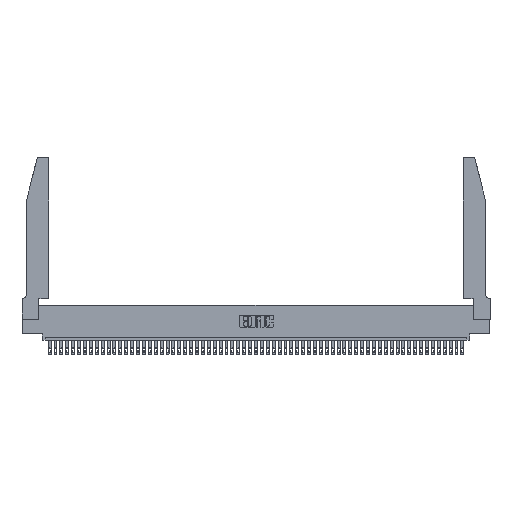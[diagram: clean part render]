
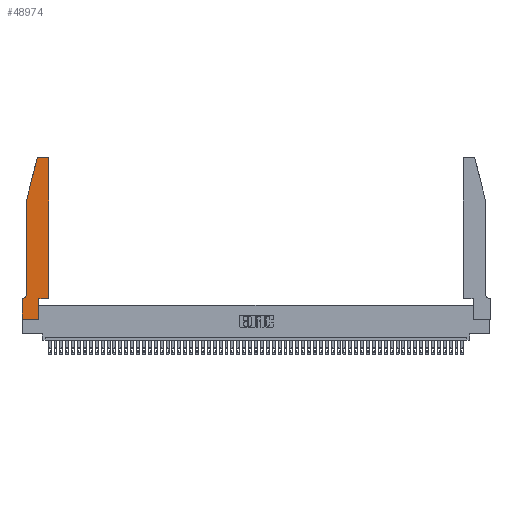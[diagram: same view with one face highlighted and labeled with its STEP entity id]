
A CAD part, top view. The second image highlights one B-rep face of the part: STEP entity #48974.
In plain terms, the highlighted planar face has unit normal (0, 0, 1).
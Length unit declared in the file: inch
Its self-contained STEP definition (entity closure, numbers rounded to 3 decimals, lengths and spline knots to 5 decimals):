
#235 = LINE ( 'NONE', #23584, #13973 ) ;
#309 = ORIENTED_EDGE ( 'NONE', *, *, #26216, .T. ) ;
#399 = LINE ( 'NONE', #14041, #47661 ) ;
#977 = EDGE_CURVE ( 'NONE', #34113, #47304, #235, .T. ) ;
#1268 = DIRECTION ( 'NONE',  ( 0., -1., 0. ) ) ;
#1806 = CIRCLE ( 'NONE', #15870, 0.07 ) ;
#2004 = DIRECTION ( 'NONE',  ( -1., 0., 0. ) ) ;
#3105 = LINE ( 'NONE', #48498, #46448 ) ;
#3688 = DIRECTION ( 'NONE',  ( 1., 0., 0. ) ) ;
#4073 = CARTESIAN_POINT ( 'NONE',  ( 0.4505, 2.72, 0.37 ) ) ;
#5131 = ORIENTED_EDGE ( 'NONE', *, *, #16956, .T. ) ;
#5728 = DIRECTION ( 'NONE',  ( 0., 0., 1. ) ) ;
#6964 = VERTEX_POINT ( 'NONE', #10926 ) ;
#7626 = ORIENTED_EDGE ( 'NONE', *, *, #21330, .T. ) ;
#7640 = EDGE_CURVE ( 'NONE', #53000, #34113, #32343, .T. ) ;
#10670 = VECTOR ( 'NONE', #36656, 39.37008 ) ;
#10926 = CARTESIAN_POINT ( 'NONE',  ( 0.0755, 0.42, 0.37 ) ) ;
#11258 = CARTESIAN_POINT ( 'NONE',  ( 0., 0., 0.37 ) ) ;
#11355 = CARTESIAN_POINT ( 'NONE',  ( 0., 0., 0.37 ) ) ;
#12174 = CARTESIAN_POINT ( 'NONE',  ( 0.4205, 2.72, 0.37 ) ) ;
#13198 = ORIENTED_EDGE ( 'NONE', *, *, #43641, .T. ) ;
#13973 = VECTOR ( 'NONE', #48124, 39.37008 ) ;
#14041 = CARTESIAN_POINT ( 'NONE',  ( 0., 0., 0.37 ) ) ;
#14532 = VECTOR ( 'NONE', #49606, 39.37008 ) ;
#15870 = AXIS2_PLACEMENT_3D ( 'NONE', #52650, #45582, #28115 ) ;
#16956 = EDGE_CURVE ( 'NONE', #47304, #45289, #17943, .T. ) ;
#17035 = ORIENTED_EDGE ( 'NONE', *, *, #7640, .T. ) ;
#17943 = LINE ( 'NONE', #32434, #42941 ) ;
#19148 = CARTESIAN_POINT ( 'NONE',  ( 0.0755, 2., 0.37 ) ) ;
#20047 = EDGE_CURVE ( 'NONE', #6964, #53029, #1806, .T. ) ;
#20269 = ORIENTED_EDGE ( 'NONE', *, *, #977, .T. ) ;
#20418 = DIRECTION ( 'NONE',  ( 1., 0., 0. ) ) ;
#20957 = CARTESIAN_POINT ( 'NONE',  ( 0., 0.35, 0.37 ) ) ;
#21146 = VECTOR ( 'NONE', #40324, 39.37008 ) ;
#21330 = EDGE_CURVE ( 'NONE', #27046, #53000, #399, .T. ) ;
#21798 = LINE ( 'NONE', #47888, #10670 ) ;
#21905 = DIRECTION ( 'NONE',  ( -0.239, -0.971, 0. ) ) ;
#23169 = CARTESIAN_POINT ( 'NONE',  ( 0.0755, 0.35, 0.37 ) ) ;
#23584 = CARTESIAN_POINT ( 'NONE',  ( 0.2865, 0.35, 0.37 ) ) ;
#24395 = CIRCLE ( 'NONE', #32426, 0.03 ) ;
#24747 = VECTOR ( 'NONE', #21905, 39.37008 ) ;
#24847 = EDGE_CURVE ( 'NONE', #53029, #27046, #38065, .T. ) ;
#25334 = VERTEX_POINT ( 'NONE', #4073 ) ;
#26216 = EDGE_CURVE ( 'NONE', #31813, #6964, #3105, .T. ) ;
#26396 = CARTESIAN_POINT ( 'NONE',  ( 0.284, 2.75, 0.37 ) ) ;
#26504 = ORIENTED_EDGE ( 'NONE', *, *, #39388, .T. ) ;
#27046 = VERTEX_POINT ( 'NONE', #34101 ) ;
#27980 = DIRECTION ( 'NONE',  ( 0., -1., 0. ) ) ;
#28115 = DIRECTION ( 'NONE',  ( -1., 0., 0. ) ) ;
#28411 = LINE ( 'NONE', #45953, #14532 ) ;
#29351 = DIRECTION ( 'NONE',  ( 0., 0., 1. ) ) ;
#30271 = CARTESIAN_POINT ( 'NONE',  ( 0.2865, 0., 0.37 ) ) ;
#30774 = ORIENTED_EDGE ( 'NONE', *, *, #41009, .T. ) ;
#31813 = VERTEX_POINT ( 'NONE', #19148 ) ;
#32343 = LINE ( 'NONE', #11355, #21146 ) ;
#32426 = AXIS2_PLACEMENT_3D ( 'NONE', #12174, #29351, #37151 ) ;
#32434 = CARTESIAN_POINT ( 'NONE',  ( 0.4505, 0.35, 0.37 ) ) ;
#34003 = AXIS2_PLACEMENT_3D ( 'NONE', #39186, #5728, #3688 ) ;
#34101 = CARTESIAN_POINT ( 'NONE',  ( 0., 0.35, 0.37 ) ) ;
#34113 = VERTEX_POINT ( 'NONE', #30271 ) ;
#34253 = CARTESIAN_POINT ( 'NONE',  ( 0.0755, 2., 0.37 ) ) ;
#36656 = DIRECTION ( 'NONE',  ( 0., 1., 0. ) ) ;
#36691 = DIRECTION ( 'NONE',  ( 1., 0., 0. ) ) ;
#37151 = DIRECTION ( 'NONE',  ( 1., 0., 0. ) ) ;
#37349 = AXIS2_PLACEMENT_3D ( 'NONE', #20957, #41367, #20418 ) ;
#37382 = PLANE ( 'NONE',  #37349 ) ;
#38065 = LINE ( 'NONE', #23169, #46530 ) ;
#38602 = VERTEX_POINT ( 'NONE', #40010 ) ;
#38679 = ORIENTED_EDGE ( 'NONE', *, *, #20047, .T. ) ;
#39127 = LINE ( 'NONE', #34253, #24747 ) ;
#39186 = CARTESIAN_POINT ( 'NONE',  ( 0.284, 2.72, 0.37 ) ) ;
#39388 = EDGE_CURVE ( 'NONE', #50389, #38602, #42034, .T. ) ;
#39435 = ORIENTED_EDGE ( 'NONE', *, *, #53190, .T. ) ;
#39783 = ORIENTED_EDGE ( 'NONE', *, *, #24847, .T. ) ;
#40010 = CARTESIAN_POINT ( 'NONE',  ( 0.25487, 2.72718, 0.37 ) ) ;
#40324 = DIRECTION ( 'NONE',  ( 1., 0., 0. ) ) ;
#41009 = EDGE_CURVE ( 'NONE', #38602, #31813, #39127, .T. ) ;
#41367 = DIRECTION ( 'NONE',  ( 0., 0., 1. ) ) ;
#42034 = CIRCLE ( 'NONE', #34003, 0.03 ) ;
#42711 = CARTESIAN_POINT ( 'NONE',  ( 0.4505, 0.35, 0.37 ) ) ;
#42941 = VECTOR ( 'NONE', #36691, 39.37008 ) ;
#43641 = EDGE_CURVE ( 'NONE', #45289, #25334, #21798, .T. ) ;
#44439 = EDGE_CURVE ( 'NONE', #25334, #51392, #24395, .T. ) ;
#45289 = VERTEX_POINT ( 'NONE', #42711 ) ;
#45582 = DIRECTION ( 'NONE',  ( 0., 0., -1. ) ) ;
#45953 = CARTESIAN_POINT ( 'NONE',  ( 0.2605, 2.75, 0.37 ) ) ;
#46448 = VECTOR ( 'NONE', #27980, 39.37008 ) ;
#46530 = VECTOR ( 'NONE', #2004, 39.37008 ) ;
#46856 = FACE_OUTER_BOUND ( 'NONE', #49076, .T. ) ;
#47270 = CARTESIAN_POINT ( 'NONE',  ( 0.4205, 2.75, 0.37 ) ) ;
#47304 = VERTEX_POINT ( 'NONE', #49512 ) ;
#47661 = VECTOR ( 'NONE', #1268, 39.37008 ) ;
#47888 = CARTESIAN_POINT ( 'NONE',  ( 0.4505, 0.35, 0.37 ) ) ;
#48124 = DIRECTION ( 'NONE',  ( 0., 1., 0. ) ) ;
#48498 = CARTESIAN_POINT ( 'NONE',  ( 0.0755, 2., 0.37 ) ) ;
#48575 = ORIENTED_EDGE ( 'NONE', *, *, #44439, .T. ) ;
#48974 = ADVANCED_FACE ( 'NONE', ( #46856 ), #37382, .T. ) ;
#49076 = EDGE_LOOP ( 'NONE', ( #39435, #26504, #30774, #309, #38679, #39783, #7626, #17035, #20269, #5131, #13198, #48575 ) ) ;
#49512 = CARTESIAN_POINT ( 'NONE',  ( 0.2865, 0.35, 0.37 ) ) ;
#49606 = DIRECTION ( 'NONE',  ( -1., 0., 0. ) ) ;
#50389 = VERTEX_POINT ( 'NONE', #26396 ) ;
#51392 = VERTEX_POINT ( 'NONE', #47270 ) ;
#52650 = CARTESIAN_POINT ( 'NONE',  ( 0.0055, 0.42, 0.37 ) ) ;
#53000 = VERTEX_POINT ( 'NONE', #11258 ) ;
#53029 = VERTEX_POINT ( 'NONE', #53269 ) ;
#53190 = EDGE_CURVE ( 'NONE', #51392, #50389, #28411, .T. ) ;
#53269 = CARTESIAN_POINT ( 'NONE',  ( 0.0055, 0.35, 0.37 ) ) ;
